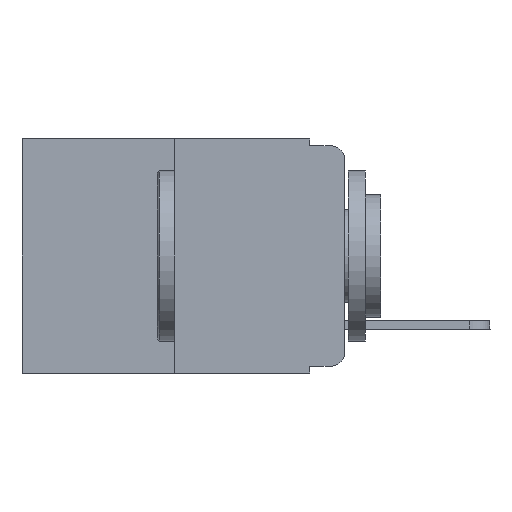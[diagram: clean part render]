
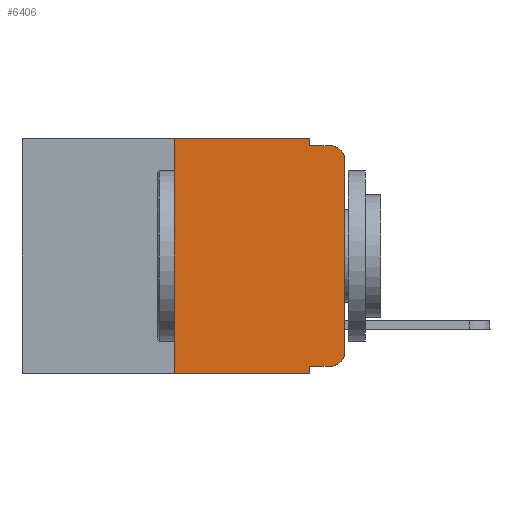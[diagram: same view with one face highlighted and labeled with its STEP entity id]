
A CAD part, left-side view. The second image highlights one B-rep face of the part: STEP entity #6406.
In plain terms, the highlighted planar face has unit normal (-1, 0, 0).
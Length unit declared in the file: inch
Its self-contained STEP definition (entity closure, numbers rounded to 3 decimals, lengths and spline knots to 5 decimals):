
#53 = CARTESIAN_POINT ( 'NONE',  ( 0., 0., 0. ) ) ;
#354 = VERTEX_POINT ( 'NONE', #9916 ) ;
#397 = DIRECTION ( 'NONE',  ( 0., -1., 0. ) ) ;
#600 = CARTESIAN_POINT ( 'NONE',  ( 0., 0.051, 0. ) ) ;
#610 = VECTOR ( 'NONE', #6533, 39.37008 ) ;
#661 = CARTESIAN_POINT ( 'NONE',  ( 0., 0.02, -0.333 ) ) ;
#1135 = ORIENTED_EDGE ( 'NONE', *, *, #2460, .F. ) ;
#1946 = EDGE_CURVE ( 'NONE', #12064, #5485, #18658, .T. ) ;
#2002 = DIRECTION ( 'NONE',  ( 1., 0., 0. ) ) ;
#2277 = EDGE_CURVE ( 'NONE', #354, #14782, #11286, .T. ) ;
#2460 = EDGE_CURVE ( 'NONE', #7080, #12064, #6001, .T. ) ;
#3230 = AXIS2_PLACEMENT_3D ( 'NONE', #13482, #22621, #11086 ) ;
#3625 = CARTESIAN_POINT ( 'NONE',  ( 0., 0.051, 0. ) ) ;
#3785 = ORIENTED_EDGE ( 'NONE', *, *, #1946, .F. ) ;
#3836 = EDGE_CURVE ( 'NONE', #10293, #12844, #11258, .T. ) ;
#3875 = LINE ( 'NONE', #18023, #10823 ) ;
#4071 = PLANE ( 'NONE',  #20656 ) ;
#4641 = DIRECTION ( 'NONE',  ( 0., 0., -1. ) ) ;
#4913 = CARTESIAN_POINT ( 'NONE',  ( 0., 0., -0.03 ) ) ;
#5059 = VECTOR ( 'NONE', #9146, 39.37008 ) ;
#5485 = VERTEX_POINT ( 'NONE', #6873 ) ;
#5519 = CARTESIAN_POINT ( 'NONE',  ( 0., 0.051, 0. ) ) ;
#5543 = LINE ( 'NONE', #3625, #18147 ) ;
#5599 = CARTESIAN_POINT ( 'NONE',  ( 0., 0.051, -0.333 ) ) ;
#5828 = VERTEX_POINT ( 'NONE', #19689 ) ;
#6001 = LINE ( 'NONE', #600, #610 ) ;
#6406 = ADVANCED_FACE ( 'NONE', ( #13959 ), #4071, .F. ) ;
#6533 = DIRECTION ( 'NONE',  ( 0., 0., -1. ) ) ;
#6854 = ORIENTED_EDGE ( 'NONE', *, *, #23007, .F. ) ;
#6873 = CARTESIAN_POINT ( 'NONE',  ( 0., 0.02, -0.01 ) ) ;
#7080 = VERTEX_POINT ( 'NONE', #5519 ) ;
#8357 = VECTOR ( 'NONE', #11413, 39.37008 ) ;
#8360 = CARTESIAN_POINT ( 'NONE',  ( 0., 0.02, -0.313 ) ) ;
#9146 = DIRECTION ( 'NONE',  ( 0., -1., 0. ) ) ;
#9365 = CARTESIAN_POINT ( 'NONE',  ( 0., 0.25, 0. ) ) ;
#9462 = DIRECTION ( 'NONE',  ( 0., -1., 0. ) ) ;
#9655 = ORIENTED_EDGE ( 'NONE', *, *, #2277, .F. ) ;
#9916 = CARTESIAN_POINT ( 'NONE',  ( 0., 0.25, -0.343 ) ) ;
#9951 = LINE ( 'NONE', #53, #21511 ) ;
#10196 = EDGE_CURVE ( 'NONE', #10293, #5828, #5543, .T. ) ;
#10293 = VERTEX_POINT ( 'NONE', #12208 ) ;
#10392 = CARTESIAN_POINT ( 'NONE',  ( 0., 0.051, -0.01 ) ) ;
#10823 = VECTOR ( 'NONE', #397, 39.37008 ) ;
#10970 = VERTEX_POINT ( 'NONE', #22930 ) ;
#11044 = CARTESIAN_POINT ( 'NONE',  ( 0., 0.473, 0. ) ) ;
#11086 = DIRECTION ( 'NONE',  ( 0., 0., -1. ) ) ;
#11168 = DIRECTION ( 'NONE',  ( 0., -1., 0. ) ) ;
#11258 = LINE ( 'NONE', #5599, #15584 ) ;
#11286 = LINE ( 'NONE', #9365, #8357 ) ;
#11413 = DIRECTION ( 'NONE',  ( 0., 0., 1. ) ) ;
#11491 = ORIENTED_EDGE ( 'NONE', *, *, #10196, .F. ) ;
#11680 = EDGE_CURVE ( 'NONE', #12844, #10970, #19428, .T. ) ;
#12064 = VERTEX_POINT ( 'NONE', #10392 ) ;
#12208 = CARTESIAN_POINT ( 'NONE',  ( 0., 0.051, -0.333 ) ) ;
#12271 = ORIENTED_EDGE ( 'NONE', *, *, #3836, .T. ) ;
#12844 = VERTEX_POINT ( 'NONE', #661 ) ;
#12965 = LINE ( 'NONE', #11044, #16589 ) ;
#13115 = ORIENTED_EDGE ( 'NONE', *, *, #18299, .T. ) ;
#13482 = CARTESIAN_POINT ( 'NONE',  ( 0., 0.02, -0.03 ) ) ;
#13959 = FACE_OUTER_BOUND ( 'NONE', #15316, .T. ) ;
#14018 = DIRECTION ( 'NONE',  ( -1., 0., 0. ) ) ;
#14782 = VERTEX_POINT ( 'NONE', #16712 ) ;
#15316 = EDGE_LOOP ( 'NONE', ( #24229, #13115, #3785, #1135, #6854, #9655, #25352, #11491, #12271, #18689 ) ) ;
#15515 = DIRECTION ( 'NONE',  ( 0., 0., -1. ) ) ;
#15584 = VECTOR ( 'NONE', #9462, 39.37008 ) ;
#15638 = CARTESIAN_POINT ( 'NONE',  ( 0., 0.473, 0. ) ) ;
#16164 = AXIS2_PLACEMENT_3D ( 'NONE', #8360, #14018, #4641 ) ;
#16589 = VECTOR ( 'NONE', #11168, 39.37008 ) ;
#16712 = CARTESIAN_POINT ( 'NONE',  ( 0., 0.25, 0. ) ) ;
#18023 = CARTESIAN_POINT ( 'NONE',  ( 0., 0.473, -0.343 ) ) ;
#18147 = VECTOR ( 'NONE', #19297, 39.37008 ) ;
#18299 = EDGE_CURVE ( 'NONE', #20843, #5485, #24976, .T. ) ;
#18658 = LINE ( 'NONE', #20575, #5059 ) ;
#18689 = ORIENTED_EDGE ( 'NONE', *, *, #11680, .T. ) ;
#19297 = DIRECTION ( 'NONE',  ( 0., 0., -1. ) ) ;
#19428 = CIRCLE ( 'NONE', #16164, 0.02 ) ;
#19689 = CARTESIAN_POINT ( 'NONE',  ( 0., 0.051, -0.343 ) ) ;
#20103 = DIRECTION ( 'NONE',  ( 0., 0., 1. ) ) ;
#20575 = CARTESIAN_POINT ( 'NONE',  ( 0., 0.051, -0.01 ) ) ;
#20656 = AXIS2_PLACEMENT_3D ( 'NONE', #15638, #2002, #15515 ) ;
#20843 = VERTEX_POINT ( 'NONE', #4913 ) ;
#21145 = EDGE_CURVE ( 'NONE', #354, #5828, #3875, .T. ) ;
#21511 = VECTOR ( 'NONE', #20103, 39.37008 ) ;
#22621 = DIRECTION ( 'NONE',  ( -1., 0., 0. ) ) ;
#22930 = CARTESIAN_POINT ( 'NONE',  ( 0., 0., -0.313 ) ) ;
#23007 = EDGE_CURVE ( 'NONE', #14782, #7080, #12965, .T. ) ;
#23756 = EDGE_CURVE ( 'NONE', #10970, #20843, #9951, .T. ) ;
#24229 = ORIENTED_EDGE ( 'NONE', *, *, #23756, .T. ) ;
#24976 = CIRCLE ( 'NONE', #3230, 0.02 ) ;
#25352 = ORIENTED_EDGE ( 'NONE', *, *, #21145, .T. ) ;
